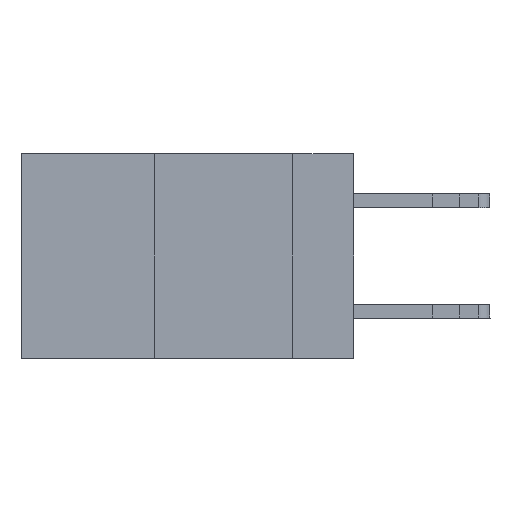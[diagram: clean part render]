
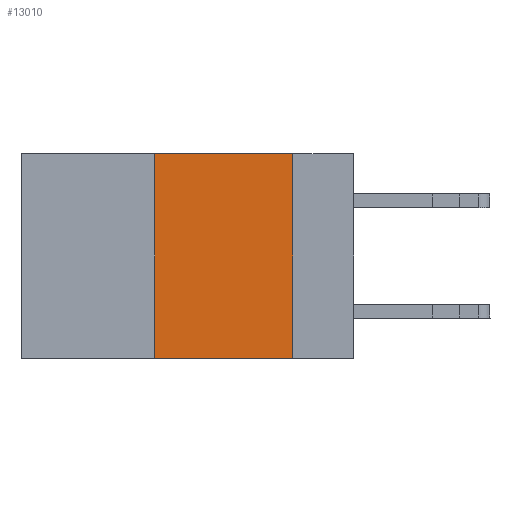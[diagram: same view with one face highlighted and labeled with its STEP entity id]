
A CAD part, left-side view. The second image highlights one B-rep face of the part: STEP entity #13010.
In plain terms, the highlighted planar face has unit normal (-1, 0, 0).
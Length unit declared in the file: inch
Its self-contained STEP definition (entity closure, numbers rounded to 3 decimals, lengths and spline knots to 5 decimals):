
#505 = VERTEX_POINT ( 'NONE', #4227 ) ;
#2518 = VECTOR ( 'NONE', #14328, 39.37008 ) ;
#3100 = CARTESIAN_POINT ( 'NONE',  ( 0., 0.6, 0. ) ) ;
#3788 = DIRECTION ( 'NONE',  ( 0., 0., 1. ) ) ;
#4227 = CARTESIAN_POINT ( 'NONE',  ( 0., 0.11, 0. ) ) ;
#4279 = LINE ( 'NONE', #16262, #2518 ) ;
#6526 = CARTESIAN_POINT ( 'NONE',  ( 0., 0.36, 0. ) ) ;
#9885 = VECTOR ( 'NONE', #19218, 39.37008 ) ;
#10755 = CARTESIAN_POINT ( 'NONE',  ( 0., 0.36, -0.37 ) ) ;
#11531 = EDGE_CURVE ( 'NONE', #15177, #20538, #4279, .T. ) ;
#11700 = CARTESIAN_POINT ( 'NONE',  ( 0., 0.36, 0. ) ) ;
#12750 = ORIENTED_EDGE ( 'NONE', *, *, #11531, .T. ) ;
#13010 = ADVANCED_FACE ( 'NONE', ( #23540 ), #21522, .F. ) ;
#14328 = DIRECTION ( 'NONE',  ( 0., -1., 0. ) ) ;
#15177 = VERTEX_POINT ( 'NONE', #10755 ) ;
#15555 = EDGE_CURVE ( 'NONE', #20411, #505, #21108, .T. ) ;
#16262 = CARTESIAN_POINT ( 'NONE',  ( 0., 0.6, -0.37 ) ) ;
#16652 = AXIS2_PLACEMENT_3D ( 'NONE', #3100, #25662, #17608 ) ;
#17608 = DIRECTION ( 'NONE',  ( 0., 0., -1. ) ) ;
#18257 = VECTOR ( 'NONE', #3788, 39.37008 ) ;
#18465 = VECTOR ( 'NONE', #24065, 39.37008 ) ;
#18489 = ORIENTED_EDGE ( 'NONE', *, *, #19717, .F. ) ;
#19218 = DIRECTION ( 'NONE',  ( 0., -1., 0. ) ) ;
#19659 = LINE ( 'NONE', #11700, #18257 ) ;
#19717 = EDGE_CURVE ( 'NONE', #505, #20538, #26330, .T. ) ;
#20411 = VERTEX_POINT ( 'NONE', #6526 ) ;
#20538 = VERTEX_POINT ( 'NONE', #23476 ) ;
#21108 = LINE ( 'NONE', #21376, #9885 ) ;
#21376 = CARTESIAN_POINT ( 'NONE',  ( 0., 0.6, 0. ) ) ;
#21522 = PLANE ( 'NONE',  #16652 ) ;
#22038 = CARTESIAN_POINT ( 'NONE',  ( 0., 0.11, 0. ) ) ;
#22553 = ORIENTED_EDGE ( 'NONE', *, *, #15555, .F. ) ;
#23273 = EDGE_LOOP ( 'NONE', ( #18489, #22553, #23908, #12750 ) ) ;
#23475 = EDGE_CURVE ( 'NONE', #15177, #20411, #19659, .T. ) ;
#23476 = CARTESIAN_POINT ( 'NONE',  ( 0., 0.11, -0.37 ) ) ;
#23540 = FACE_OUTER_BOUND ( 'NONE', #23273, .T. ) ;
#23908 = ORIENTED_EDGE ( 'NONE', *, *, #23475, .F. ) ;
#24065 = DIRECTION ( 'NONE',  ( 0., 0., -1. ) ) ;
#25662 = DIRECTION ( 'NONE',  ( 1., 0., 0. ) ) ;
#26330 = LINE ( 'NONE', #22038, #18465 ) ;
